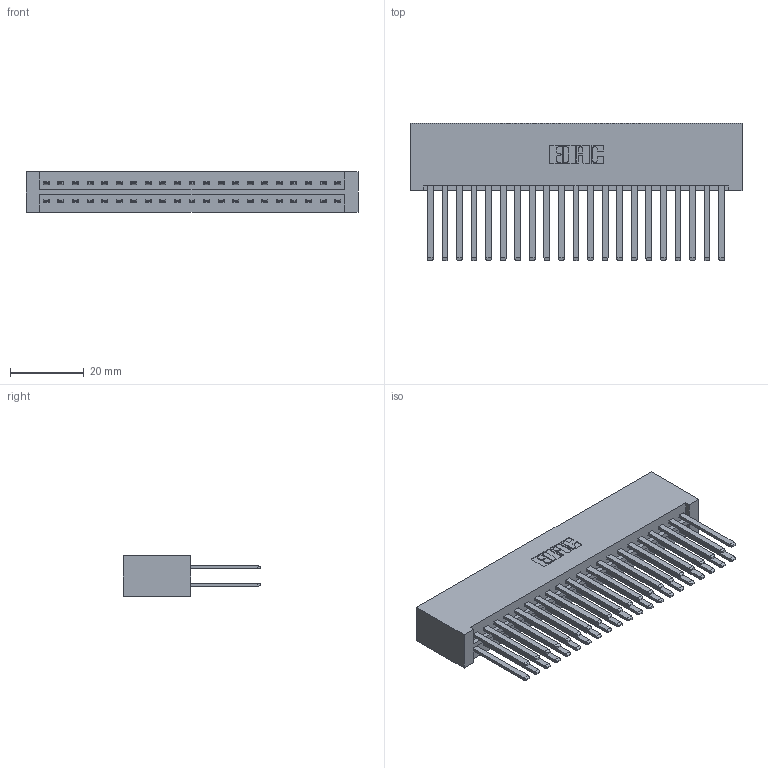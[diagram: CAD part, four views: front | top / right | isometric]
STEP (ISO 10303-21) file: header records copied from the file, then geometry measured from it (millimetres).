
FILE_DESCRIPTION (( 'STEP AP203' ), '1' );
FILE_NAME ('336-042-541-801.STEP', '2020-08-07T23:37:23', ( '' ), ( '' ), 'SwSTEP 2.0', 'SolidWorks 2020', '' );
FILE_SCHEMA (( 'CONFIG_CONTROL_DESIGN' ));
Length unit declared in the file: inch
Products named in the file (3): 336 Part_Lugless; 336-042-541-801; 336-290-001_336-290-541
Assembly tree (43 placements, depth 2):
  336-042-541-801
    336 Part_Lugless
    336-290-001_336-290-541  x42
Bounding box: 90.32 x 37.34 x 11.1 mm (x, y, z)
Volume: 14940.5 mm3; surface area: 18862.1 mm2
Topology: 43 solids, 43 shells, 1870 faces, 5621 edges, 3718 vertices
Faces by surface type: plane 1158, cylinder 712
Entity records: 18440 total; most frequent: CARTESIAN_POINT 3205, ORIENTED_EDGE 3042, DIRECTION 2661, EDGE_CURVE 1521, LINE 1397, VECTOR 1397, VERTEX_POINT 1012, AXIS2_PLACEMENT_3D 632
